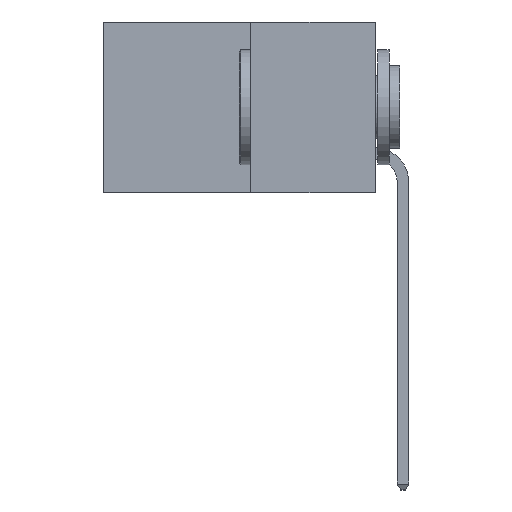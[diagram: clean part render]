
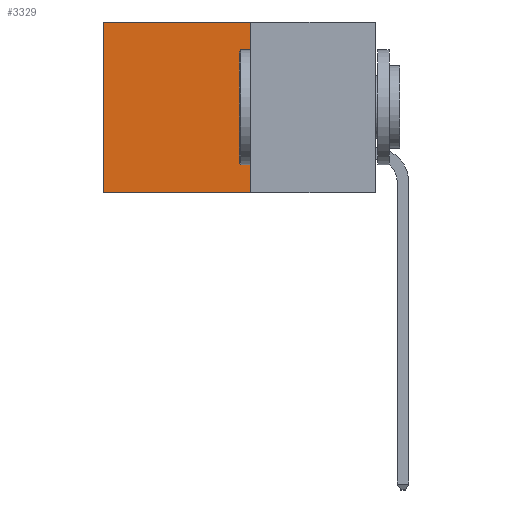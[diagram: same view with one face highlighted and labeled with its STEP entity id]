
A CAD part, left-side view. The second image highlights one B-rep face of the part: STEP entity #3329.
In plain terms, the highlighted planar face has unit normal (-1, 0, 0).
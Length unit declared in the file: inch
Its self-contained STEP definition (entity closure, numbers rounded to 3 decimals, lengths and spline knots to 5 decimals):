
#9 = CARTESIAN_POINT ( 'NONE',  ( 0.277, 0.27, -0.37 ) ) ;
#969 = FACE_OUTER_BOUND ( 'NONE', #10265, .T. ) ;
#1094 = VECTOR ( 'NONE', #9617, 39.37008 ) ;
#1590 = ORIENTED_EDGE ( 'NONE', *, *, #5288, .T. ) ;
#3213 = CARTESIAN_POINT ( 'NONE',  ( 0.277, 0.27, -0.37 ) ) ;
#3329 = ADVANCED_FACE ( 'NONE', ( #969 ), #7420, .F. ) ;
#3532 = LINE ( 'NONE', #9, #5936 ) ;
#3581 = LINE ( 'NONE', #4312, #8746 ) ;
#3660 = DIRECTION ( 'NONE',  ( 0., 0., -1. ) ) ;
#4094 = LINE ( 'NONE', #14732, #13444 ) ;
#4291 = DIRECTION ( 'NONE',  ( 0., 0., -1. ) ) ;
#4312 = CARTESIAN_POINT ( 'NONE',  ( 0.277, 0.59, -0.37 ) ) ;
#4315 = VERTEX_POINT ( 'NONE', #14638 ) ;
#4341 = AXIS2_PLACEMENT_3D ( 'NONE', #7598, #7369, #7330 ) ;
#4789 = ORIENTED_EDGE ( 'NONE', *, *, #6040, .F. ) ;
#5288 = EDGE_CURVE ( 'NONE', #4315, #6377, #3581, .T. ) ;
#5811 = CARTESIAN_POINT ( 'NONE',  ( 0.277, 0.27, 0. ) ) ;
#5936 = VECTOR ( 'NONE', #3660, 39.37008 ) ;
#6040 = EDGE_CURVE ( 'NONE', #9612, #6377, #13280, .T. ) ;
#6377 = VERTEX_POINT ( 'NONE', #15082 ) ;
#6691 = EDGE_CURVE ( 'NONE', #14916, #4315, #4094, .T. ) ;
#7027 = DIRECTION ( 'NONE',  ( 0., 1., 0. ) ) ;
#7330 = DIRECTION ( 'NONE',  ( 0., 0., -1. ) ) ;
#7369 = DIRECTION ( 'NONE',  ( 1., 0., 0. ) ) ;
#7420 = PLANE ( 'NONE',  #4341 ) ;
#7598 = CARTESIAN_POINT ( 'NONE',  ( 0.277, 0.27, -0.37 ) ) ;
#8454 = CARTESIAN_POINT ( 'NONE',  ( 0.277, 0.27, -0.37 ) ) ;
#8746 = VECTOR ( 'NONE', #4291, 39.37008 ) ;
#9612 = VERTEX_POINT ( 'NONE', #3213 ) ;
#9617 = DIRECTION ( 'NONE',  ( 0., 1., 0. ) ) ;
#10265 = EDGE_LOOP ( 'NONE', ( #1590, #4789, #11036, #14087 ) ) ;
#10323 = EDGE_CURVE ( 'NONE', #14916, #9612, #3532, .T. ) ;
#11036 = ORIENTED_EDGE ( 'NONE', *, *, #10323, .F. ) ;
#13280 = LINE ( 'NONE', #8454, #1094 ) ;
#13444 = VECTOR ( 'NONE', #7027, 39.37008 ) ;
#14087 = ORIENTED_EDGE ( 'NONE', *, *, #6691, .T. ) ;
#14638 = CARTESIAN_POINT ( 'NONE',  ( 0.277, 0.59, 0. ) ) ;
#14732 = CARTESIAN_POINT ( 'NONE',  ( 0.277, 0.27, 0. ) ) ;
#14916 = VERTEX_POINT ( 'NONE', #5811 ) ;
#15082 = CARTESIAN_POINT ( 'NONE',  ( 0.277, 0.59, -0.37 ) ) ;
